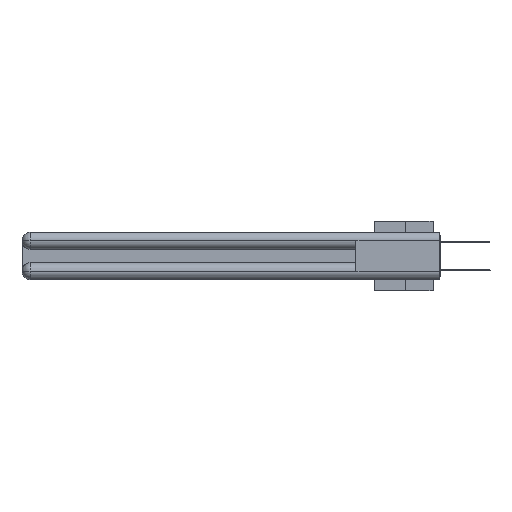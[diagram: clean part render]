
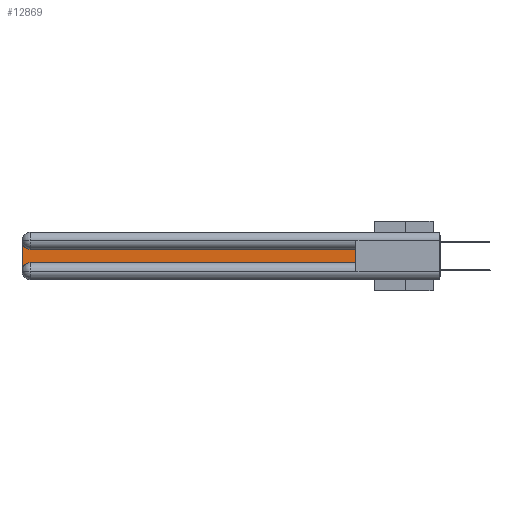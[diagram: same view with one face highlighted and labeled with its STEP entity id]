
A CAD part, left-side view. The second image highlights one B-rep face of the part: STEP entity #12869.
In plain terms, the highlighted planar face has unit normal (-1, 0, 0).
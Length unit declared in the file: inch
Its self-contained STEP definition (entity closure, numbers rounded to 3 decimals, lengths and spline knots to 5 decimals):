
#1020 = LINE ( 'NONE', #3764, #2829 ) ;
#1126 = CARTESIAN_POINT ( 'NONE',  ( 0.075, 3., -0.0625 ) ) ;
#1130 = VECTOR ( 'NONE', #7569, 39.37008 ) ;
#2422 = CARTESIAN_POINT ( 'NONE',  ( 0.075, 2.94, -0.0625 ) ) ;
#2768 = CARTESIAN_POINT ( 'NONE',  ( 0.075, 2.94, -0.2175 ) ) ;
#2829 = VECTOR ( 'NONE', #15511, 39.37008 ) ;
#3305 = VERTEX_POINT ( 'NONE', #1126 ) ;
#3476 = EDGE_CURVE ( 'NONE', #23065, #17233, #36509, .T. ) ;
#3764 = CARTESIAN_POINT ( 'NONE',  ( 0.075, 3., -0.2175 ) ) ;
#3965 = EDGE_CURVE ( 'NONE', #17233, #3305, #5760, .T. ) ;
#5760 = CIRCLE ( 'NONE', #30655, 0.06 ) ;
#5899 = EDGE_LOOP ( 'NONE', ( #21866, #20014, #15074, #7825, #20866, #33135 ) ) ;
#6206 = EDGE_CURVE ( 'NONE', #29649, #8168, #35482, .T. ) ;
#7346 = CARTESIAN_POINT ( 'NONE',  ( 0.075, 3., -0.2775 ) ) ;
#7569 = DIRECTION ( 'NONE',  ( 0., 0., 1. ) ) ;
#7825 = ORIENTED_EDGE ( 'NONE', *, *, #29379, .T. ) ;
#7844 = EDGE_CURVE ( 'NONE', #3305, #23665, #1020, .T. ) ;
#8107 = AXIS2_PLACEMENT_3D ( 'NONE', #34870, #18305, #21154 ) ;
#8112 = DIRECTION ( 'NONE',  ( 0., 1., 0. ) ) ;
#8168 = VERTEX_POINT ( 'NONE', #9694 ) ;
#9240 = CIRCLE ( 'NONE', #15210, 0.06 ) ;
#9694 = CARTESIAN_POINT ( 'NONE',  ( 0.075, 0.6, -0.2175 ) ) ;
#10659 = DIRECTION ( 'NONE',  ( 0., 0., -1. ) ) ;
#12567 = CARTESIAN_POINT ( 'NONE',  ( 0.075, 2.94, -0.1225 ) ) ;
#12869 = ADVANCED_FACE ( 'NONE', ( #20806 ), #15436, .F. ) ;
#13412 = DIRECTION ( 'NONE',  ( 1., 0., 0. ) ) ;
#15074 = ORIENTED_EDGE ( 'NONE', *, *, #7844, .T. ) ;
#15210 = AXIS2_PLACEMENT_3D ( 'NONE', #35540, #35790, #24343 ) ;
#15436 = PLANE ( 'NONE',  #8107 ) ;
#15511 = DIRECTION ( 'NONE',  ( 0., 0., -1. ) ) ;
#16817 = DIRECTION ( 'NONE',  ( 0., -1., 0. ) ) ;
#17233 = VERTEX_POINT ( 'NONE', #12567 ) ;
#18305 = DIRECTION ( 'NONE',  ( 1., 0., 0. ) ) ;
#19404 = LINE ( 'NONE', #22498, #1130 ) ;
#20014 = ORIENTED_EDGE ( 'NONE', *, *, #3965, .T. ) ;
#20806 = FACE_OUTER_BOUND ( 'NONE', #5899, .T. ) ;
#20866 = ORIENTED_EDGE ( 'NONE', *, *, #6206, .T. ) ;
#21154 = DIRECTION ( 'NONE',  ( 0., 0., -1. ) ) ;
#21866 = ORIENTED_EDGE ( 'NONE', *, *, #3476, .T. ) ;
#22498 = CARTESIAN_POINT ( 'NONE',  ( 0.075, 0.6, -0.2175 ) ) ;
#23065 = VERTEX_POINT ( 'NONE', #35903 ) ;
#23665 = VERTEX_POINT ( 'NONE', #7346 ) ;
#24343 = DIRECTION ( 'NONE',  ( 0., 0., -1. ) ) ;
#25433 = CARTESIAN_POINT ( 'NONE',  ( 0.075, 0.6, -0.1225 ) ) ;
#25708 = VECTOR ( 'NONE', #16817, 39.37008 ) ;
#28938 = VECTOR ( 'NONE', #8112, 39.37008 ) ;
#29379 = EDGE_CURVE ( 'NONE', #23665, #29649, #9240, .T. ) ;
#29649 = VERTEX_POINT ( 'NONE', #2768 ) ;
#30655 = AXIS2_PLACEMENT_3D ( 'NONE', #2422, #13412, #10659 ) ;
#30805 = EDGE_CURVE ( 'NONE', #8168, #23065, #19404, .T. ) ;
#33135 = ORIENTED_EDGE ( 'NONE', *, *, #30805, .T. ) ;
#33899 = CARTESIAN_POINT ( 'NONE',  ( 0.075, 0.6, -0.2175 ) ) ;
#34870 = CARTESIAN_POINT ( 'NONE',  ( 0.075, 3., -0.1225 ) ) ;
#35482 = LINE ( 'NONE', #33899, #25708 ) ;
#35540 = CARTESIAN_POINT ( 'NONE',  ( 0.075, 2.94, -0.2775 ) ) ;
#35790 = DIRECTION ( 'NONE',  ( 1., 0., 0. ) ) ;
#35903 = CARTESIAN_POINT ( 'NONE',  ( 0.075, 0.6, -0.1225 ) ) ;
#36509 = LINE ( 'NONE', #25433, #28938 ) ;
